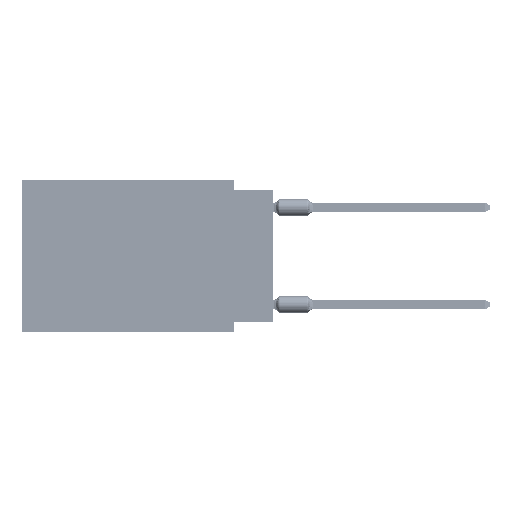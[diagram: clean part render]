
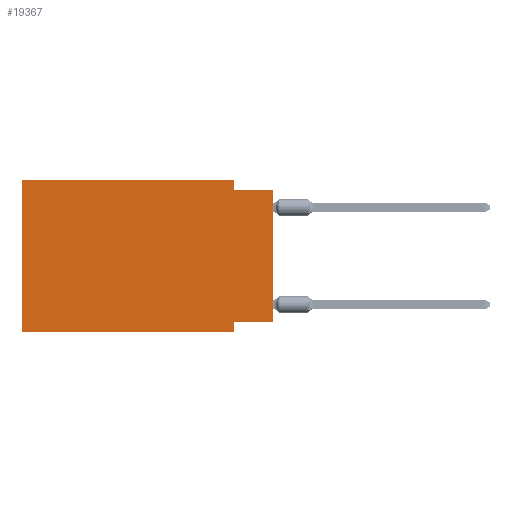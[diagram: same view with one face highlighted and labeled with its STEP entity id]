
A CAD part, left-side view. The second image highlights one B-rep face of the part: STEP entity #19367.
In plain terms, the highlighted planar face has unit normal (-1, 0, 0).
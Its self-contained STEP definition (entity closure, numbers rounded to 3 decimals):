
#794 = PLANE ( 'NONE',  #42462 ) ;
#1279 = ORIENTED_EDGE ( 'NONE', *, *, #51987, .F. ) ;
#4791 = DIRECTION ( 'NONE',  ( 0., -1., 0. ) ) ;
#5481 = ORIENTED_EDGE ( 'NONE', *, *, #67726, .F. ) ;
#6764 = DIRECTION ( 'NONE',  ( 0., 0., 1. ) ) ;
#6804 = ORIENTED_EDGE ( 'NONE', *, *, #33306, .F. ) ;
#6901 = DIRECTION ( 'NONE',  ( 0., 1., 0. ) ) ;
#8235 = EDGE_CURVE ( 'NONE', #43184, #72469, #57848, .T. ) ;
#10923 = CARTESIAN_POINT ( 'NONE',  ( 0., 16.383, -9.906 ) ) ;
#11990 = CARTESIAN_POINT ( 'NONE',  ( 0., 0., -9.271 ) ) ;
#14968 = VECTOR ( 'NONE', #21091, 1000. ) ;
#16176 = CARTESIAN_POINT ( 'NONE',  ( 0., 2.54, -0.635 ) ) ;
#16457 = CARTESIAN_POINT ( 'NONE',  ( 0., 0., 0. ) ) ;
#17356 = DIRECTION ( 'NONE',  ( 0., -1., 0. ) ) ;
#18785 = DIRECTION ( 'NONE',  ( 1., 0., 0. ) ) ;
#19367 = ADVANCED_FACE ( 'NONE', ( #58774 ), #794, .F. ) ;
#19641 = ORIENTED_EDGE ( 'NONE', *, *, #8235, .F. ) ;
#20182 = VERTEX_POINT ( 'NONE', #49836 ) ;
#21091 = DIRECTION ( 'NONE',  ( 0., -1., 0. ) ) ;
#22619 = CARTESIAN_POINT ( 'NONE',  ( 0., 16.383, 0. ) ) ;
#23061 = EDGE_LOOP ( 'NONE', ( #72474, #69412, #19641, #57227, #1279, #77299, #5481, #6804 ) ) ;
#24361 = CARTESIAN_POINT ( 'NONE',  ( 0., 16.383, 0. ) ) ;
#25599 = CARTESIAN_POINT ( 'NONE',  ( 0., 2.54, -9.906 ) ) ;
#28133 = VERTEX_POINT ( 'NONE', #66217 ) ;
#30031 = VERTEX_POINT ( 'NONE', #70020 ) ;
#33306 = EDGE_CURVE ( 'NONE', #20182, #30031, #66019, .T. ) ;
#33312 = LINE ( 'NONE', #16457, #41600 ) ;
#33608 = LINE ( 'NONE', #68886, #14968 ) ;
#33973 = VERTEX_POINT ( 'NONE', #10923 ) ;
#36572 = LINE ( 'NONE', #25599, #49914 ) ;
#38627 = CARTESIAN_POINT ( 'NONE',  ( 0., 2.54, 0. ) ) ;
#38833 = DIRECTION ( 'NONE',  ( 0., 0., 1. ) ) ;
#41244 = VECTOR ( 'NONE', #17356, 1000. ) ;
#41600 = VECTOR ( 'NONE', #38833, 1000. ) ;
#42462 = AXIS2_PLACEMENT_3D ( 'NONE', #43868, #18785, #42704 ) ;
#42704 = DIRECTION ( 'NONE',  ( 0., 0., -1. ) ) ;
#43184 = VERTEX_POINT ( 'NONE', #38627 ) ;
#43868 = CARTESIAN_POINT ( 'NONE',  ( 0., 16.383, 0. ) ) ;
#45200 = EDGE_CURVE ( 'NONE', #72469, #28133, #58822, .T. ) ;
#47570 = VERTEX_POINT ( 'NONE', #69657 ) ;
#49139 = EDGE_CURVE ( 'NONE', #33973, #47570, #33608, .T. ) ;
#49836 = CARTESIAN_POINT ( 'NONE',  ( 0., 0., -9.271 ) ) ;
#49914 = VECTOR ( 'NONE', #54608, 1000. ) ;
#51406 = CARTESIAN_POINT ( 'NONE',  ( 0., 0., -0.635 ) ) ;
#51535 = VECTOR ( 'NONE', #6764, 1000. ) ;
#51987 = EDGE_CURVE ( 'NONE', #33973, #52870, #65882, .T. ) ;
#52353 = EDGE_CURVE ( 'NONE', #20182, #28133, #33312, .T. ) ;
#52870 = VERTEX_POINT ( 'NONE', #22619 ) ;
#53796 = LINE ( 'NONE', #59275, #41244 ) ;
#54608 = DIRECTION ( 'NONE',  ( 0., 0., -1. ) ) ;
#55183 = EDGE_CURVE ( 'NONE', #52870, #43184, #53796, .T. ) ;
#57227 = ORIENTED_EDGE ( 'NONE', *, *, #55183, .F. ) ;
#57848 = LINE ( 'NONE', #59001, #75771 ) ;
#58774 = FACE_OUTER_BOUND ( 'NONE', #23061, .T. ) ;
#58822 = LINE ( 'NONE', #51406, #67321 ) ;
#59001 = CARTESIAN_POINT ( 'NONE',  ( 0., 2.54, 0. ) ) ;
#59275 = CARTESIAN_POINT ( 'NONE',  ( 0., 16.383, 0. ) ) ;
#60466 = VECTOR ( 'NONE', #6901, 1000. ) ;
#65882 = LINE ( 'NONE', #24361, #51535 ) ;
#66019 = LINE ( 'NONE', #11990, #60466 ) ;
#66217 = CARTESIAN_POINT ( 'NONE',  ( 0., 0., -0.635 ) ) ;
#67321 = VECTOR ( 'NONE', #4791, 1000. ) ;
#67726 = EDGE_CURVE ( 'NONE', #30031, #47570, #36572, .T. ) ;
#68886 = CARTESIAN_POINT ( 'NONE',  ( 0., 16.383, -9.906 ) ) ;
#69412 = ORIENTED_EDGE ( 'NONE', *, *, #45200, .F. ) ;
#69657 = CARTESIAN_POINT ( 'NONE',  ( 0., 2.54, -9.906 ) ) ;
#70020 = CARTESIAN_POINT ( 'NONE',  ( 0., 2.54, -9.271 ) ) ;
#72469 = VERTEX_POINT ( 'NONE', #16176 ) ;
#72474 = ORIENTED_EDGE ( 'NONE', *, *, #52353, .T. ) ;
#75771 = VECTOR ( 'NONE', #76267, 1000. ) ;
#76267 = DIRECTION ( 'NONE',  ( 0., 0., -1. ) ) ;
#77299 = ORIENTED_EDGE ( 'NONE', *, *, #49139, .T. ) ;
